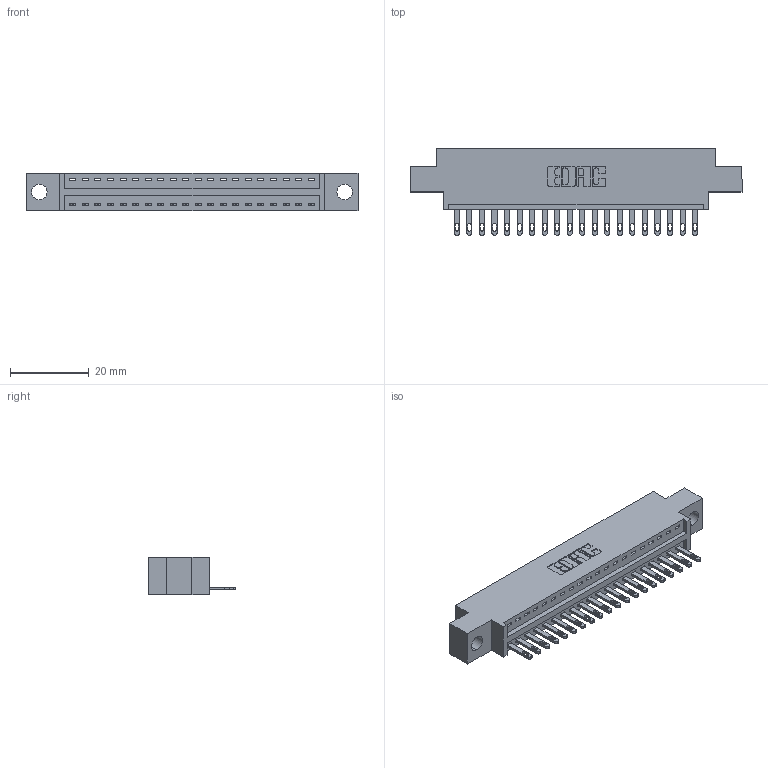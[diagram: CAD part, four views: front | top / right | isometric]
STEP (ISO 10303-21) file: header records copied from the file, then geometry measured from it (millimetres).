
FILE_DESCRIPTION (( 'STEP AP203' ), '1' );
FILE_NAME ('346-020-500-604.STEP', '2022-05-05T16:07:25', ( '' ), ( '' ), 'SwSTEP 2.0', 'SolidWorks 2020', '' );
FILE_SCHEMA (( 'CONFIG_CONTROL_DESIGN' ));
Length unit declared in the file: inch
Products named in the file (3): 346-020-500-604; 345-292-001_345-293-100; 346 Part_0.170 Offset - 0.156 Dia-TH
Assembly tree (21 placements, depth 2):
  346-020-500-604
    346 Part_0.170 Offset - 0.156 Dia-TH
    345-292-001_345-293-100  x20
Bounding box: 84.07 x 21.84 x 9.4 mm (x, y, z)
Volume: 7648 mm3; surface area: 9365.8 mm2
Topology: 21 solids, 21 shells, 1220 faces, 3737 edges, 2490 vertices
Faces by surface type: plane 774, cylinder 446
Entity records: 15855 total; most frequent: CARTESIAN_POINT 2734, ORIENTED_EDGE 2686, DIRECTION 2439, EDGE_CURVE 1343, VECTOR 1127, LINE 1127, VERTEX_POINT 894, AXIS2_PLACEMENT_3D 656
